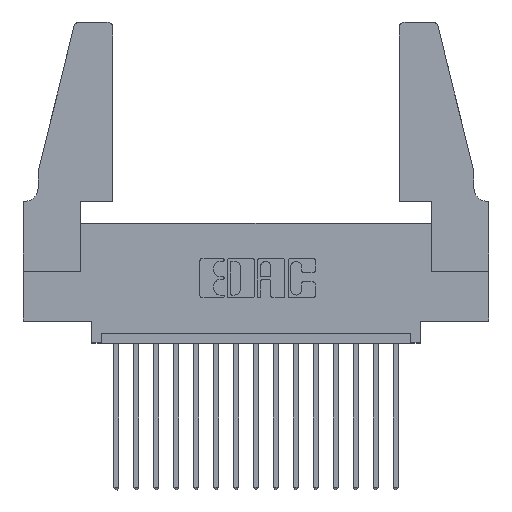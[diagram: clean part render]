
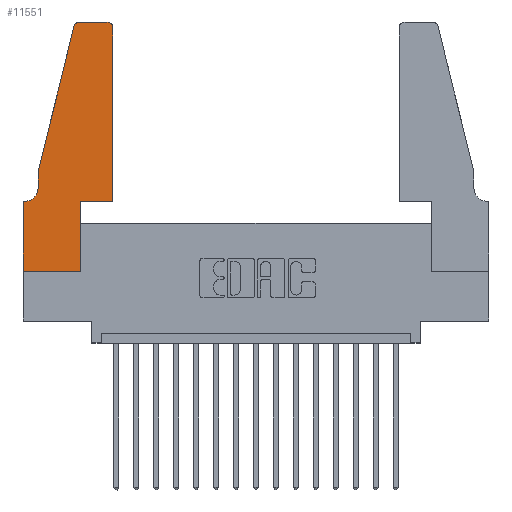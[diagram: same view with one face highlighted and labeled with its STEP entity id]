
A CAD part, top view. The second image highlights one B-rep face of the part: STEP entity #11551.
In plain terms, the highlighted planar face has unit normal (0, 0, 1).
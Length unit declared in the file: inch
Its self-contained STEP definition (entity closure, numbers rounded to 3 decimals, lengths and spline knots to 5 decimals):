
#288 = CIRCLE ( 'NONE', #8544, 0.07 ) ;
#400 = VECTOR ( 'NONE', #2958, 39.37008 ) ;
#803 = EDGE_CURVE ( 'NONE', #14176, #2023, #15093, .T. ) ;
#858 = DIRECTION ( 'NONE',  ( 1., 0., 0. ) ) ;
#944 = VECTOR ( 'NONE', #1447, 39.37008 ) ;
#1000 = VERTEX_POINT ( 'NONE', #7453 ) ;
#1280 = CARTESIAN_POINT ( 'NONE',  ( 0.4205, 1.22, 0.37 ) ) ;
#1414 = VERTEX_POINT ( 'NONE', #12541 ) ;
#1447 = DIRECTION ( 'NONE',  ( -1., 0., 0. ) ) ;
#1471 = LINE ( 'NONE', #2294, #8962 ) ;
#1928 = LINE ( 'NONE', #3129, #12746 ) ;
#2023 = VERTEX_POINT ( 'NONE', #3483 ) ;
#2101 = VERTEX_POINT ( 'NONE', #9944 ) ;
#2294 = CARTESIAN_POINT ( 'NONE',  ( 0., 0., 0.37 ) ) ;
#2393 = DIRECTION ( 'NONE',  ( -1., 0., 0. ) ) ;
#2492 = CARTESIAN_POINT ( 'NONE',  ( 0.0755, 0.42, 0.37 ) ) ;
#2871 = AXIS2_PLACEMENT_3D ( 'NONE', #1280, #3853, #9189 ) ;
#2958 = DIRECTION ( 'NONE',  ( 0., -1., 0. ) ) ;
#3008 = VECTOR ( 'NONE', #6956, 39.37008 ) ;
#3129 = CARTESIAN_POINT ( 'NONE',  ( 0.2865, 0.35, 0.37 ) ) ;
#3226 = CARTESIAN_POINT ( 'NONE',  ( 0.0755, 0.35, 0.37 ) ) ;
#3318 = LINE ( 'NONE', #13661, #400 ) ;
#3483 = CARTESIAN_POINT ( 'NONE',  ( 0.284, 1.25, 0.37 ) ) ;
#3533 = EDGE_CURVE ( 'NONE', #13705, #1000, #1471, .T. ) ;
#3761 = VECTOR ( 'NONE', #8042, 39.37008 ) ;
#3853 = DIRECTION ( 'NONE',  ( 0., 0., 1. ) ) ;
#3960 = EDGE_CURVE ( 'NONE', #11395, #2101, #13955, .T. ) ;
#4194 = CARTESIAN_POINT ( 'NONE',  ( 0.4205, 1.25, 0.37 ) ) ;
#4257 = CIRCLE ( 'NONE', #5440, 0.03 ) ;
#4449 = CARTESIAN_POINT ( 'NONE',  ( 0.2865, 0.35, 0.37 ) ) ;
#4590 = VERTEX_POINT ( 'NONE', #6503 ) ;
#5030 = CARTESIAN_POINT ( 'NONE',  ( 0.4505, 0.35, 0.37 ) ) ;
#5161 = LINE ( 'NONE', #3226, #9102 ) ;
#5440 = AXIS2_PLACEMENT_3D ( 'NONE', #15634, #12939, #13002 ) ;
#5486 = CARTESIAN_POINT ( 'NONE',  ( 0.2605, 1.25, 0.37 ) ) ;
#5726 = ORIENTED_EDGE ( 'NONE', *, *, #9427, .T. ) ;
#5978 = EDGE_CURVE ( 'NONE', #9991, #11395, #6265, .T. ) ;
#6226 = ORIENTED_EDGE ( 'NONE', *, *, #3533, .T. ) ;
#6265 = LINE ( 'NONE', #5030, #11479 ) ;
#6503 = CARTESIAN_POINT ( 'NONE',  ( 0.0755, 0.5, 0.37 ) ) ;
#6726 = CARTESIAN_POINT ( 'NONE',  ( 0.4505, 0.35, 0.37 ) ) ;
#6956 = DIRECTION ( 'NONE',  ( -0.239, -0.971, 0. ) ) ;
#7013 = EDGE_CURVE ( 'NONE', #4590, #16890, #3318, .T. ) ;
#7073 = DIRECTION ( 'NONE',  ( 1., 0., 0. ) ) ;
#7392 = ORIENTED_EDGE ( 'NONE', *, *, #10985, .T. ) ;
#7453 = CARTESIAN_POINT ( 'NONE',  ( 0., 0., 0.37 ) ) ;
#7629 = EDGE_CURVE ( 'NONE', #1414, #13705, #5161, .T. ) ;
#7885 = CARTESIAN_POINT ( 'NONE',  ( 0.25487, 1.22718, 0.37 ) ) ;
#7940 = ORIENTED_EDGE ( 'NONE', *, *, #3960, .T. ) ;
#8042 = DIRECTION ( 'NONE',  ( 0., 1., 0. ) ) ;
#8544 = AXIS2_PLACEMENT_3D ( 'NONE', #16445, #11885, #2393 ) ;
#8946 = CARTESIAN_POINT ( 'NONE',  ( 0.2865, 0., 0.37 ) ) ;
#8962 = VECTOR ( 'NONE', #12941, 39.37008 ) ;
#8979 = ORIENTED_EDGE ( 'NONE', *, *, #7629, .T. ) ;
#9087 = VERTEX_POINT ( 'NONE', #7885 ) ;
#9102 = VECTOR ( 'NONE', #16255, 39.37008 ) ;
#9189 = DIRECTION ( 'NONE',  ( 1., 0., 0. ) ) ;
#9230 = EDGE_LOOP ( 'NONE', ( #14716, #12283, #5726, #14538, #14808, #8979, #6226, #13691, #7392, #10457, #7940, #10789 ) ) ;
#9427 = EDGE_CURVE ( 'NONE', #9087, #4590, #16131, .T. ) ;
#9453 = EDGE_CURVE ( 'NONE', #1000, #16804, #13830, .T. ) ;
#9516 = CARTESIAN_POINT ( 'NONE',  ( 0., 0.35, 0.37 ) ) ;
#9750 = EDGE_CURVE ( 'NONE', #2101, #14176, #10510, .T. ) ;
#9839 = CARTESIAN_POINT ( 'NONE',  ( 0.0755, 0.5, 0.37 ) ) ;
#9867 = EDGE_CURVE ( 'NONE', #16890, #1414, #288, .T. ) ;
#9944 = CARTESIAN_POINT ( 'NONE',  ( 0.4505, 1.22, 0.37 ) ) ;
#9991 = VERTEX_POINT ( 'NONE', #4449 ) ;
#10290 = CARTESIAN_POINT ( 'NONE',  ( 0., 0.35, 0.37 ) ) ;
#10457 = ORIENTED_EDGE ( 'NONE', *, *, #5978, .T. ) ;
#10510 = CIRCLE ( 'NONE', #2871, 0.03 ) ;
#10789 = ORIENTED_EDGE ( 'NONE', *, *, #9750, .T. ) ;
#10985 = EDGE_CURVE ( 'NONE', #16804, #9991, #1928, .T. ) ;
#11039 = DIRECTION ( 'NONE',  ( 0., 1., 0. ) ) ;
#11123 = VECTOR ( 'NONE', #7073, 39.37008 ) ;
#11395 = VERTEX_POINT ( 'NONE', #13954 ) ;
#11479 = VECTOR ( 'NONE', #14329, 39.37008 ) ;
#11551 = ADVANCED_FACE ( 'NONE', ( #15694 ), #12722, .T. ) ;
#11885 = DIRECTION ( 'NONE',  ( 0., 0., -1. ) ) ;
#12283 = ORIENTED_EDGE ( 'NONE', *, *, #15070, .T. ) ;
#12541 = CARTESIAN_POINT ( 'NONE',  ( 0.0055, 0.35, 0.37 ) ) ;
#12722 = PLANE ( 'NONE',  #15639 ) ;
#12746 = VECTOR ( 'NONE', #11039, 39.37008 ) ;
#12939 = DIRECTION ( 'NONE',  ( 0., 0., 1. ) ) ;
#12941 = DIRECTION ( 'NONE',  ( 0., -1., 0. ) ) ;
#13002 = DIRECTION ( 'NONE',  ( 1., 0., 0. ) ) ;
#13570 = CARTESIAN_POINT ( 'NONE',  ( 0., 0., 0.37 ) ) ;
#13661 = CARTESIAN_POINT ( 'NONE',  ( 0.0755, 0.5, 0.37 ) ) ;
#13691 = ORIENTED_EDGE ( 'NONE', *, *, #9453, .T. ) ;
#13705 = VERTEX_POINT ( 'NONE', #9516 ) ;
#13830 = LINE ( 'NONE', #13570, #11123 ) ;
#13955 = LINE ( 'NONE', #6726, #3761 ) ;
#13954 = CARTESIAN_POINT ( 'NONE',  ( 0.4505, 0.35, 0.37 ) ) ;
#14176 = VERTEX_POINT ( 'NONE', #4194 ) ;
#14299 = DIRECTION ( 'NONE',  ( 0., 0., 1. ) ) ;
#14329 = DIRECTION ( 'NONE',  ( 1., 0., 0. ) ) ;
#14538 = ORIENTED_EDGE ( 'NONE', *, *, #7013, .T. ) ;
#14716 = ORIENTED_EDGE ( 'NONE', *, *, #803, .T. ) ;
#14808 = ORIENTED_EDGE ( 'NONE', *, *, #9867, .T. ) ;
#15070 = EDGE_CURVE ( 'NONE', #2023, #9087, #4257, .T. ) ;
#15093 = LINE ( 'NONE', #5486, #944 ) ;
#15634 = CARTESIAN_POINT ( 'NONE',  ( 0.284, 1.22, 0.37 ) ) ;
#15639 = AXIS2_PLACEMENT_3D ( 'NONE', #10290, #14299, #858 ) ;
#15694 = FACE_OUTER_BOUND ( 'NONE', #9230, .T. ) ;
#16131 = LINE ( 'NONE', #9839, #3008 ) ;
#16255 = DIRECTION ( 'NONE',  ( -1., 0., 0. ) ) ;
#16445 = CARTESIAN_POINT ( 'NONE',  ( 0.0055, 0.42, 0.37 ) ) ;
#16804 = VERTEX_POINT ( 'NONE', #8946 ) ;
#16890 = VERTEX_POINT ( 'NONE', #2492 ) ;
